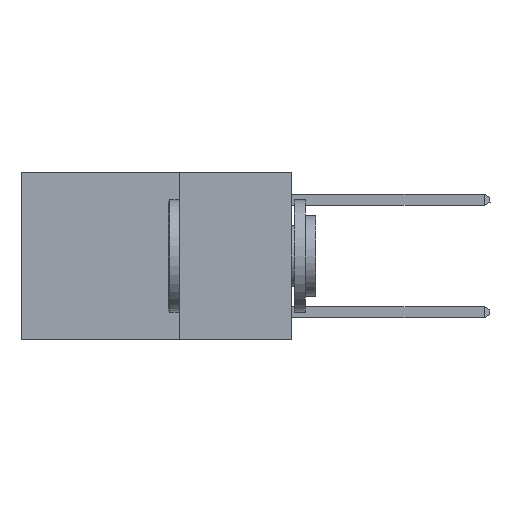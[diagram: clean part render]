
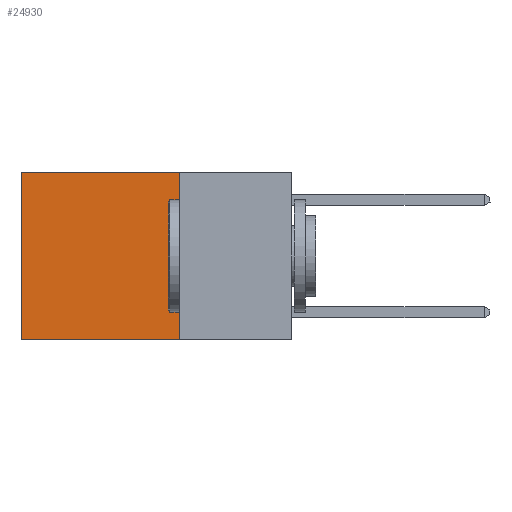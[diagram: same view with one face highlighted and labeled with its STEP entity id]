
A CAD part, left-side view. The second image highlights one B-rep face of the part: STEP entity #24930.
In plain terms, the highlighted planar face has unit normal (-1, 0, 0).
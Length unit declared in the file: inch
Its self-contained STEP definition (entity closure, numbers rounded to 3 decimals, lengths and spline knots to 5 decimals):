
#157 = VERTEX_POINT ( 'NONE', #8890 ) ;
#2486 = EDGE_CURVE ( 'NONE', #27002, #157, #7018, .T. ) ;
#2789 = DIRECTION ( 'NONE',  ( 0., 1., 0. ) ) ;
#3004 = ORIENTED_EDGE ( 'NONE', *, *, #2486, .T. ) ;
#3534 = LINE ( 'NONE', #18994, #27960 ) ;
#4051 = FACE_OUTER_BOUND ( 'NONE', #17186, .T. ) ;
#4161 = DIRECTION ( 'NONE',  ( 0., 0., -1. ) ) ;
#4634 = ORIENTED_EDGE ( 'NONE', *, *, #23479, .T. ) ;
#6624 = AXIS2_PLACEMENT_3D ( 'NONE', #13050, #29423, #11021 ) ;
#7018 = LINE ( 'NONE', #18226, #23493 ) ;
#8890 = CARTESIAN_POINT ( 'NONE',  ( 0.2625, 0.6, -0.37 ) ) ;
#10143 = ORIENTED_EDGE ( 'NONE', *, *, #11604, .F. ) ;
#10918 = VERTEX_POINT ( 'NONE', #29439 ) ;
#10929 = LINE ( 'NONE', #26346, #14163 ) ;
#11021 = DIRECTION ( 'NONE',  ( 0., 0., -1. ) ) ;
#11604 = EDGE_CURVE ( 'NONE', #27205, #157, #10929, .T. ) ;
#13050 = CARTESIAN_POINT ( 'NONE',  ( 0.2625, 0.25, 0. ) ) ;
#14163 = VECTOR ( 'NONE', #2789, 39.37008 ) ;
#16908 = ORIENTED_EDGE ( 'NONE', *, *, #19407, .F. ) ;
#17186 = EDGE_LOOP ( 'NONE', ( #3004, #10143, #16908, #4634 ) ) ;
#18226 = CARTESIAN_POINT ( 'NONE',  ( 0.2625, 0.6, 0. ) ) ;
#18806 = LINE ( 'NONE', #21259, #20265 ) ;
#18994 = CARTESIAN_POINT ( 'NONE',  ( 0.2625, 0.25, 0. ) ) ;
#19407 = EDGE_CURVE ( 'NONE', #10918, #27205, #3534, .T. ) ;
#20265 = VECTOR ( 'NONE', #27538, 39.37008 ) ;
#20700 = DIRECTION ( 'NONE',  ( 0., 0., -1. ) ) ;
#21259 = CARTESIAN_POINT ( 'NONE',  ( 0.2625, 0.25, 0. ) ) ;
#22550 = CARTESIAN_POINT ( 'NONE',  ( 0.2625, 0.6, 0. ) ) ;
#23479 = EDGE_CURVE ( 'NONE', #10918, #27002, #18806, .T. ) ;
#23493 = VECTOR ( 'NONE', #4161, 39.37008 ) ;
#24192 = CARTESIAN_POINT ( 'NONE',  ( 0.2625, 0.25, -0.37 ) ) ;
#24930 = ADVANCED_FACE ( 'NONE', ( #4051 ), #24953, .F. ) ;
#24953 = PLANE ( 'NONE',  #6624 ) ;
#26346 = CARTESIAN_POINT ( 'NONE',  ( 0.2625, 0.25, -0.37 ) ) ;
#27002 = VERTEX_POINT ( 'NONE', #22550 ) ;
#27205 = VERTEX_POINT ( 'NONE', #24192 ) ;
#27538 = DIRECTION ( 'NONE',  ( 0., 1., 0. ) ) ;
#27960 = VECTOR ( 'NONE', #20700, 39.37008 ) ;
#29423 = DIRECTION ( 'NONE',  ( 1., 0., 0. ) ) ;
#29439 = CARTESIAN_POINT ( 'NONE',  ( 0.2625, 0.25, 0. ) ) ;
